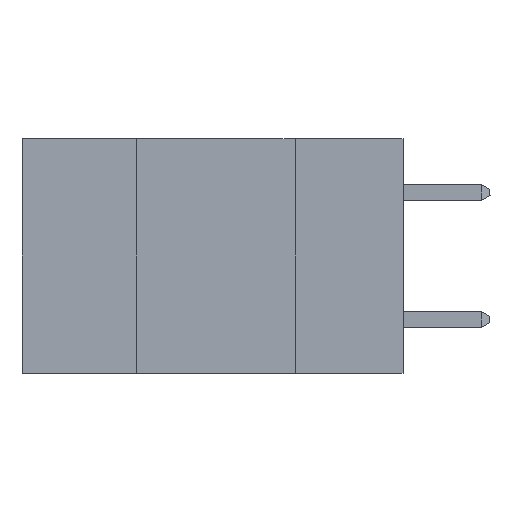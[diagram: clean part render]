
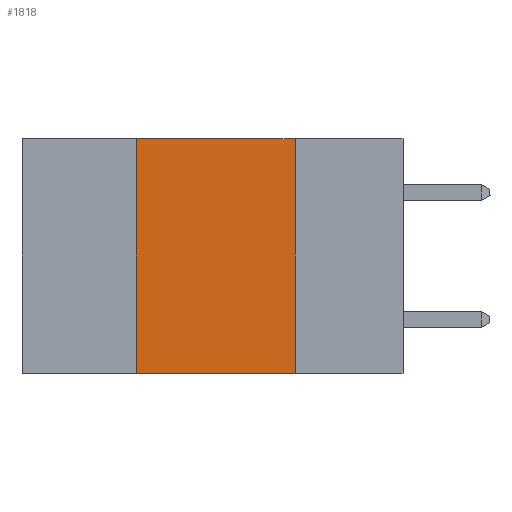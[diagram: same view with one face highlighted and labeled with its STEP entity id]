
A CAD part, left-side view. The second image highlights one B-rep face of the part: STEP entity #1818.
In plain terms, the highlighted planar face has unit normal (-1, 0, 0).
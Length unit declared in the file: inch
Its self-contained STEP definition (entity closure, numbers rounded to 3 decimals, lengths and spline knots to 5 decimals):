
#238 = ORIENTED_EDGE ( 'NONE', *, *, #5380, .F. ) ;
#365 = CARTESIAN_POINT ( 'NONE',  ( 0., 0.17, 0. ) ) ;
#708 = CARTESIAN_POINT ( 'NONE',  ( 0., 0.17, 0. ) ) ;
#1488 = CARTESIAN_POINT ( 'NONE',  ( 0., 0.6, -0.37 ) ) ;
#1727 = CARTESIAN_POINT ( 'NONE',  ( 0., 0.42, 0. ) ) ;
#1760 = EDGE_LOOP ( 'NONE', ( #15913, #238, #23913, #23653 ) ) ;
#1818 = ADVANCED_FACE ( 'NONE', ( #22884 ), #23952, .F. ) ;
#1900 = VERTEX_POINT ( 'NONE', #708 ) ;
#2423 = VECTOR ( 'NONE', #17207, 39.37008 ) ;
#3486 = DIRECTION ( 'NONE',  ( 0., -1., 0. ) ) ;
#3713 = DIRECTION ( 'NONE',  ( 0., 0., 1. ) ) ;
#3754 = VERTEX_POINT ( 'NONE', #22938 ) ;
#4552 = VERTEX_POINT ( 'NONE', #16597 ) ;
#5380 = EDGE_CURVE ( 'NONE', #11214, #1900, #19823, .T. ) ;
#5461 = LINE ( 'NONE', #1488, #20726 ) ;
#8135 = DIRECTION ( 'NONE',  ( 1., 0., 0. ) ) ;
#11214 = VERTEX_POINT ( 'NONE', #20557 ) ;
#12199 = VECTOR ( 'NONE', #3713, 39.37008 ) ;
#13244 = LINE ( 'NONE', #365, #18756 ) ;
#14366 = DIRECTION ( 'NONE',  ( 0., 0., -1. ) ) ;
#15877 = DIRECTION ( 'NONE',  ( 0., 0., -1. ) ) ;
#15913 = ORIENTED_EDGE ( 'NONE', *, *, #18842, .F. ) ;
#16597 = CARTESIAN_POINT ( 'NONE',  ( 0., 0.42, -0.37 ) ) ;
#17207 = DIRECTION ( 'NONE',  ( 0., -1., 0. ) ) ;
#18756 = VECTOR ( 'NONE', #14366, 39.37008 ) ;
#18842 = EDGE_CURVE ( 'NONE', #1900, #3754, #13244, .T. ) ;
#19823 = LINE ( 'NONE', #24847, #2423 ) ;
#19857 = LINE ( 'NONE', #1727, #12199 ) ;
#20171 = CARTESIAN_POINT ( 'NONE',  ( 0., 0.6, 0. ) ) ;
#20557 = CARTESIAN_POINT ( 'NONE',  ( 0., 0.42, 0. ) ) ;
#20726 = VECTOR ( 'NONE', #3486, 39.37008 ) ;
#21099 = AXIS2_PLACEMENT_3D ( 'NONE', #20171, #8135, #15877 ) ;
#21719 = EDGE_CURVE ( 'NONE', #4552, #11214, #19857, .T. ) ;
#22405 = EDGE_CURVE ( 'NONE', #4552, #3754, #5461, .T. ) ;
#22884 = FACE_OUTER_BOUND ( 'NONE', #1760, .T. ) ;
#22938 = CARTESIAN_POINT ( 'NONE',  ( 0., 0.17, -0.37 ) ) ;
#23653 = ORIENTED_EDGE ( 'NONE', *, *, #22405, .T. ) ;
#23913 = ORIENTED_EDGE ( 'NONE', *, *, #21719, .F. ) ;
#23952 = PLANE ( 'NONE',  #21099 ) ;
#24847 = CARTESIAN_POINT ( 'NONE',  ( 0., 0.6, 0. ) ) ;
